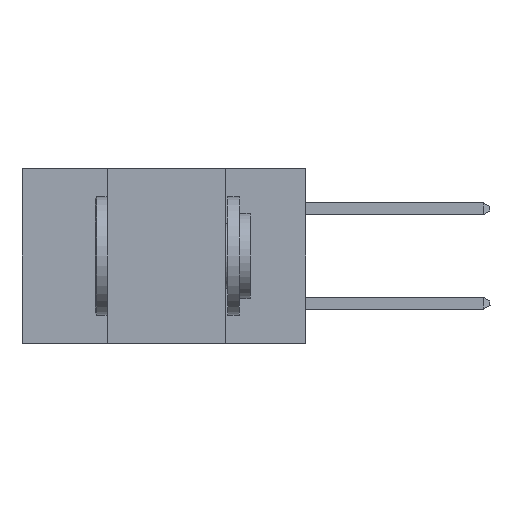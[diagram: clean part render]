
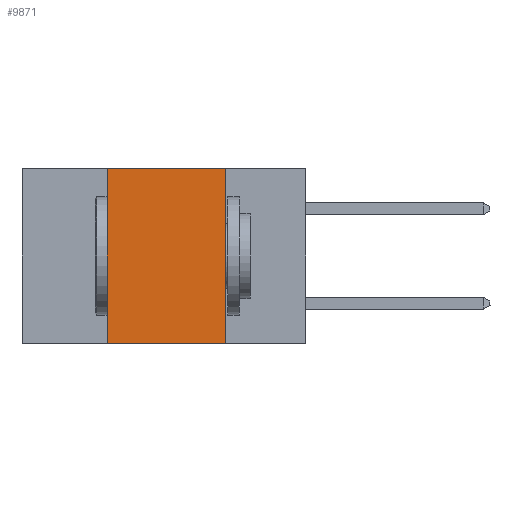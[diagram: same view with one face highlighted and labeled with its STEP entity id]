
A CAD part, left-side view. The second image highlights one B-rep face of the part: STEP entity #9871.
In plain terms, the highlighted planar face has unit normal (-1, 0, 0).
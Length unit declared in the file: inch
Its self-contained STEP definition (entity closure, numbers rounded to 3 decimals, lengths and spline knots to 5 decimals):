
#231 = EDGE_LOOP ( 'NONE', ( #1987, #3179, #1425, #6009 ) ) ;
#350 = VERTEX_POINT ( 'NONE', #10020 ) ;
#443 = DIRECTION ( 'NONE',  ( 0., -1., 0. ) ) ;
#637 = VECTOR ( 'NONE', #5772, 39.37008 ) ;
#883 = LINE ( 'NONE', #6754, #996 ) ;
#996 = VECTOR ( 'NONE', #7698, 39.37008 ) ;
#1199 = EDGE_CURVE ( 'NONE', #2350, #350, #7624, .T. ) ;
#1425 = ORIENTED_EDGE ( 'NONE', *, *, #9021, .F. ) ;
#1686 = CARTESIAN_POINT ( 'NONE',  ( 0., 0.17, -0.37 ) ) ;
#1765 = VERTEX_POINT ( 'NONE', #2623 ) ;
#1987 = ORIENTED_EDGE ( 'NONE', *, *, #4780, .F. ) ;
#2126 = LINE ( 'NONE', #1686, #7511 ) ;
#2350 = VERTEX_POINT ( 'NONE', #2904 ) ;
#2623 = CARTESIAN_POINT ( 'NONE',  ( 0., 0.17, 0. ) ) ;
#2904 = CARTESIAN_POINT ( 'NONE',  ( 0., 0.42, -0.37 ) ) ;
#2940 = FACE_OUTER_BOUND ( 'NONE', #231, .T. ) ;
#3179 = ORIENTED_EDGE ( 'NONE', *, *, #10478, .F. ) ;
#4184 = DIRECTION ( 'NONE',  ( 0., 0., -1. ) ) ;
#4780 = EDGE_CURVE ( 'NONE', #1765, #350, #2126, .T. ) ;
#5334 = LINE ( 'NONE', #10803, #637 ) ;
#5544 = DIRECTION ( 'NONE',  ( 0., 0., -1. ) ) ;
#5772 = DIRECTION ( 'NONE',  ( 0., 0., 1. ) ) ;
#6009 = ORIENTED_EDGE ( 'NONE', *, *, #1199, .T. ) ;
#6637 = VERTEX_POINT ( 'NONE', #7832 ) ;
#6754 = CARTESIAN_POINT ( 'NONE',  ( 0., 0.6, 0. ) ) ;
#6776 = AXIS2_PLACEMENT_3D ( 'NONE', #9762, #10613, #5544 ) ;
#7204 = CARTESIAN_POINT ( 'NONE',  ( 0., 0.6, -0.37 ) ) ;
#7511 = VECTOR ( 'NONE', #4184, 39.37008 ) ;
#7624 = LINE ( 'NONE', #7204, #9209 ) ;
#7698 = DIRECTION ( 'NONE',  ( 0., -1., 0. ) ) ;
#7832 = CARTESIAN_POINT ( 'NONE',  ( 0., 0.42, 0. ) ) ;
#8922 = PLANE ( 'NONE',  #6776 ) ;
#9021 = EDGE_CURVE ( 'NONE', #2350, #6637, #5334, .T. ) ;
#9209 = VECTOR ( 'NONE', #443, 39.37008 ) ;
#9762 = CARTESIAN_POINT ( 'NONE',  ( 0., 0.6, 0. ) ) ;
#9871 = ADVANCED_FACE ( 'NONE', ( #2940 ), #8922, .F. ) ;
#10020 = CARTESIAN_POINT ( 'NONE',  ( 0., 0.17, -0.37 ) ) ;
#10478 = EDGE_CURVE ( 'NONE', #6637, #1765, #883, .T. ) ;
#10613 = DIRECTION ( 'NONE',  ( 1., 0., 0. ) ) ;
#10803 = CARTESIAN_POINT ( 'NONE',  ( 0., 0.42, -0.37 ) ) ;
